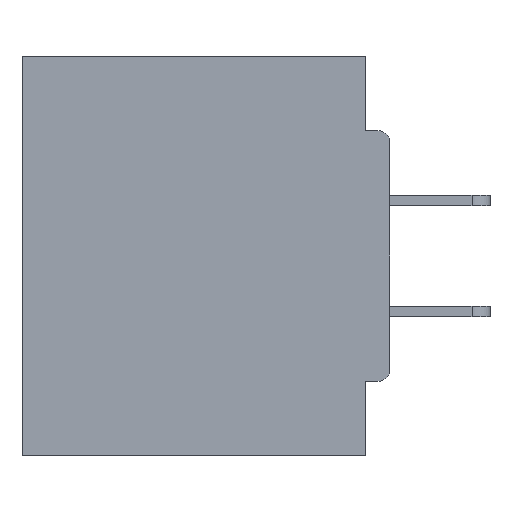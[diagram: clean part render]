
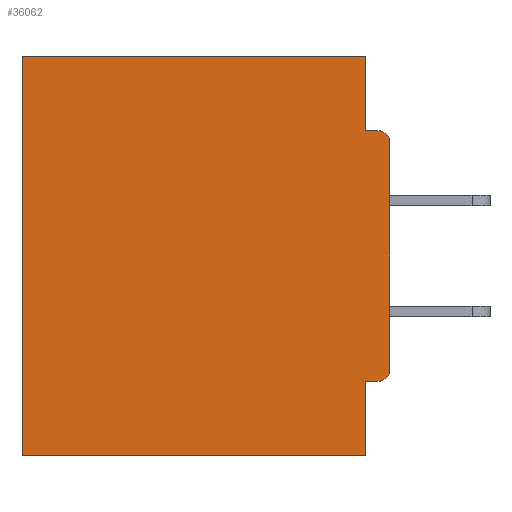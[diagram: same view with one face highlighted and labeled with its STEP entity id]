
A CAD part, left-side view. The second image highlights one B-rep face of the part: STEP entity #36062.
In plain terms, the highlighted planar face has unit normal (-1, 0, 0).
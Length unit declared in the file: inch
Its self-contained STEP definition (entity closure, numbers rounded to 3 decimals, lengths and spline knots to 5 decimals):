
#383 = VERTEX_POINT ( 'NONE', #1025 ) ;
#600 = CARTESIAN_POINT ( 'NONE',  ( 0.298, 0.031, -0.5 ) ) ;
#630 = LINE ( 'NONE', #600, #33386 ) ;
#656 = EDGE_CURVE ( 'NONE', #45168, #7453, #33534, .T. ) ;
#1025 = CARTESIAN_POINT ( 'NONE',  ( 0.298, 0.031, 0. ) ) ;
#1349 = CARTESIAN_POINT ( 'NONE',  ( 0.298, 0., 0. ) ) ;
#1388 = VECTOR ( 'NONE', #32570, 39.37008 ) ;
#1438 = DIRECTION ( 'NONE',  ( 0., -1., 0. ) ) ;
#1691 = AXIS2_PLACEMENT_3D ( 'NONE', #37432, #26715, #5480 ) ;
#3384 = VECTOR ( 'NONE', #32339, 39.37008 ) ;
#3489 = CARTESIAN_POINT ( 'NONE',  ( 0.298, 0.015, -0.1085 ) ) ;
#4279 = CARTESIAN_POINT ( 'NONE',  ( 0.298, 0., 0. ) ) ;
#4548 = CARTESIAN_POINT ( 'NONE',  ( 0.298, 0.015, -0.4065 ) ) ;
#5120 = CARTESIAN_POINT ( 'NONE',  ( 0.298, 0., -0.0935 ) ) ;
#5386 = VERTEX_POINT ( 'NONE', #14779 ) ;
#5480 = DIRECTION ( 'NONE',  ( 0., 0., -1. ) ) ;
#5861 = LINE ( 'NONE', #14846, #1388 ) ;
#6282 = EDGE_CURVE ( 'NONE', #44056, #7453, #6610, .T. ) ;
#6610 = LINE ( 'NONE', #34761, #13009 ) ;
#6686 = LINE ( 'NONE', #5120, #35579 ) ;
#7415 = DIRECTION ( 'NONE',  ( 0., 0., -1. ) ) ;
#7453 = VERTEX_POINT ( 'NONE', #37578 ) ;
#8570 = VECTOR ( 'NONE', #32123, 39.37008 ) ;
#9700 = VERTEX_POINT ( 'NONE', #4548 ) ;
#10098 = DIRECTION ( 'NONE',  ( 0., 0., -1. ) ) ;
#10514 = VERTEX_POINT ( 'NONE', #21313 ) ;
#10624 = EDGE_CURVE ( 'NONE', #383, #5386, #32241, .T. ) ;
#10638 = ORIENTED_EDGE ( 'NONE', *, *, #42907, .F. ) ;
#10949 = PLANE ( 'NONE',  #14949 ) ;
#12161 = AXIS2_PLACEMENT_3D ( 'NONE', #3489, #42454, #39022 ) ;
#13009 = VECTOR ( 'NONE', #10098, 39.37008 ) ;
#14267 = CARTESIAN_POINT ( 'NONE',  ( 0.298, 0., -0.5 ) ) ;
#14754 = ORIENTED_EDGE ( 'NONE', *, *, #24597, .T. ) ;
#14779 = CARTESIAN_POINT ( 'NONE',  ( 0.298, 0.031, -0.0935 ) ) ;
#14846 = CARTESIAN_POINT ( 'NONE',  ( 0.298, 0., -0.4065 ) ) ;
#14949 = AXIS2_PLACEMENT_3D ( 'NONE', #4279, #29059, #18046 ) ;
#15360 = ORIENTED_EDGE ( 'NONE', *, *, #39803, .F. ) ;
#15889 = ORIENTED_EDGE ( 'NONE', *, *, #29850, .F. ) ;
#18046 = DIRECTION ( 'NONE',  ( 0., 0., -1. ) ) ;
#18962 = ORIENTED_EDGE ( 'NONE', *, *, #10624, .F. ) ;
#21313 = CARTESIAN_POINT ( 'NONE',  ( 0.298, 0.015, -0.0935 ) ) ;
#21615 = CARTESIAN_POINT ( 'NONE',  ( 0.298, 0.031, -0.5 ) ) ;
#21954 = VERTEX_POINT ( 'NONE', #26733 ) ;
#21995 = ORIENTED_EDGE ( 'NONE', *, *, #6282, .T. ) ;
#22682 = CARTESIAN_POINT ( 'NONE',  ( 0.298, 0.031, -0.5 ) ) ;
#23376 = EDGE_LOOP ( 'NONE', ( #35878, #15889, #18962, #14754, #21995, #45588, #10638, #35970, #24341, #15360 ) ) ;
#24341 = ORIENTED_EDGE ( 'NONE', *, *, #29410, .T. ) ;
#24597 = EDGE_CURVE ( 'NONE', #383, #44056, #29735, .T. ) ;
#25466 = EDGE_CURVE ( 'NONE', #9700, #26045, #5861, .T. ) ;
#26045 = VERTEX_POINT ( 'NONE', #40584 ) ;
#26715 = DIRECTION ( 'NONE',  ( -1., 0., 0. ) ) ;
#26733 = CARTESIAN_POINT ( 'NONE',  ( 0.298, 0., -0.1085 ) ) ;
#27750 = DIRECTION ( 'NONE',  ( 0., 1., 0. ) ) ;
#29059 = DIRECTION ( 'NONE',  ( 1., 0., 0. ) ) ;
#29153 = LINE ( 'NONE', #1349, #29700 ) ;
#29410 = EDGE_CURVE ( 'NONE', #9700, #32892, #30591, .T. ) ;
#29700 = VECTOR ( 'NONE', #33280, 39.37008 ) ;
#29735 = LINE ( 'NONE', #34326, #45337 ) ;
#29850 = EDGE_CURVE ( 'NONE', #5386, #10514, #6686, .T. ) ;
#30591 = CIRCLE ( 'NONE', #1691, 0.015 ) ;
#32123 = DIRECTION ( 'NONE',  ( 0., 1., 0. ) ) ;
#32241 = LINE ( 'NONE', #21615, #3384 ) ;
#32339 = DIRECTION ( 'NONE',  ( 0., 0., -1. ) ) ;
#32570 = DIRECTION ( 'NONE',  ( 0., 1., 0. ) ) ;
#32892 = VERTEX_POINT ( 'NONE', #38233 ) ;
#33280 = DIRECTION ( 'NONE',  ( 0., 0., -1. ) ) ;
#33386 = VECTOR ( 'NONE', #7415, 39.37008 ) ;
#33534 = LINE ( 'NONE', #14267, #8570 ) ;
#34326 = CARTESIAN_POINT ( 'NONE',  ( 0.298, 0., 0. ) ) ;
#34761 = CARTESIAN_POINT ( 'NONE',  ( 0.298, 0.46, 0. ) ) ;
#35579 = VECTOR ( 'NONE', #1438, 39.37008 ) ;
#35878 = ORIENTED_EDGE ( 'NONE', *, *, #39519, .T. ) ;
#35970 = ORIENTED_EDGE ( 'NONE', *, *, #25466, .F. ) ;
#36062 = ADVANCED_FACE ( 'NONE', ( #42155 ), #10949, .F. ) ;
#37432 = CARTESIAN_POINT ( 'NONE',  ( 0.298, 0.015, -0.3915 ) ) ;
#37578 = CARTESIAN_POINT ( 'NONE',  ( 0.298, 0.46, -0.5 ) ) ;
#38233 = CARTESIAN_POINT ( 'NONE',  ( 0.298, 0., -0.3915 ) ) ;
#39022 = DIRECTION ( 'NONE',  ( 0., 0., -1. ) ) ;
#39519 = EDGE_CURVE ( 'NONE', #21954, #10514, #45348, .T. ) ;
#39803 = EDGE_CURVE ( 'NONE', #21954, #32892, #29153, .T. ) ;
#40584 = CARTESIAN_POINT ( 'NONE',  ( 0.298, 0.031, -0.4065 ) ) ;
#42155 = FACE_OUTER_BOUND ( 'NONE', #23376, .T. ) ;
#42454 = DIRECTION ( 'NONE',  ( -1., 0., 0. ) ) ;
#42907 = EDGE_CURVE ( 'NONE', #26045, #45168, #630, .T. ) ;
#43197 = CARTESIAN_POINT ( 'NONE',  ( 0.298, 0.46, 0. ) ) ;
#44056 = VERTEX_POINT ( 'NONE', #43197 ) ;
#45168 = VERTEX_POINT ( 'NONE', #22682 ) ;
#45337 = VECTOR ( 'NONE', #27750, 39.37008 ) ;
#45348 = CIRCLE ( 'NONE', #12161, 0.015 ) ;
#45588 = ORIENTED_EDGE ( 'NONE', *, *, #656, .F. ) ;
